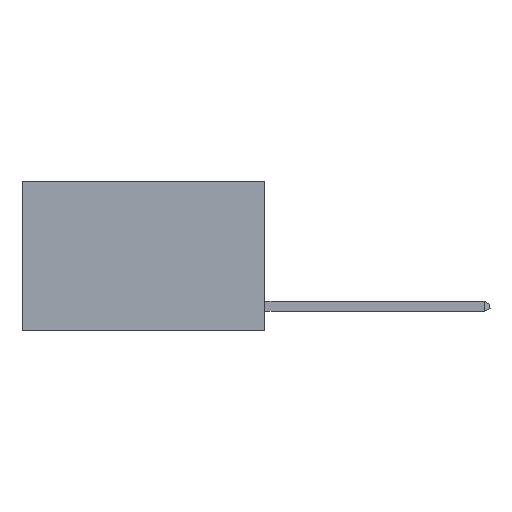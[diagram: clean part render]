
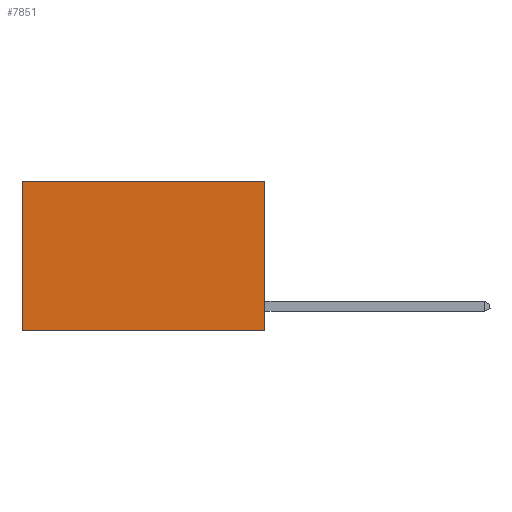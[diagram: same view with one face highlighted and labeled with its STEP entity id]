
A CAD part, left-side view. The second image highlights one B-rep face of the part: STEP entity #7851.
In plain terms, the highlighted planar face has unit normal (-1, 0, 0).
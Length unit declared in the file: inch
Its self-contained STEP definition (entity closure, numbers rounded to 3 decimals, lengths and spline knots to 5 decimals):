
#441 = LINE ( 'NONE', #6357, #4153 ) ;
#710 = ORIENTED_EDGE ( 'NONE', *, *, #3343, .F. ) ;
#729 = ORIENTED_EDGE ( 'NONE', *, *, #4248, .F. ) ;
#936 = CARTESIAN_POINT ( 'NONE',  ( 0.2625, 0., 0. ) ) ;
#1063 = CARTESIAN_POINT ( 'NONE',  ( 0.2625, 0.6, -0.37 ) ) ;
#1352 = DIRECTION ( 'NONE',  ( 0., 0., -1. ) ) ;
#1630 = VERTEX_POINT ( 'NONE', #7407 ) ;
#2320 = VECTOR ( 'NONE', #1352, 39.37008 ) ;
#2380 = DIRECTION ( 'NONE',  ( 0., 0., -1. ) ) ;
#2469 = LINE ( 'NONE', #3936, #7798 ) ;
#2563 = EDGE_CURVE ( 'NONE', #3820, #7483, #6559, .T. ) ;
#3313 = LINE ( 'NONE', #5901, #2320 ) ;
#3343 = EDGE_CURVE ( 'NONE', #3820, #1630, #3313, .T. ) ;
#3380 = CARTESIAN_POINT ( 'NONE',  ( 0.2625, 0., 0. ) ) ;
#3624 = EDGE_CURVE ( 'NONE', #7483, #3974, #441, .T. ) ;
#3820 = VERTEX_POINT ( 'NONE', #936 ) ;
#3936 = CARTESIAN_POINT ( 'NONE',  ( 0.2625, 0., -0.37 ) ) ;
#3944 = DIRECTION ( 'NONE',  ( 0., 1., 0. ) ) ;
#3974 = VERTEX_POINT ( 'NONE', #1063 ) ;
#4153 = VECTOR ( 'NONE', #7576, 39.37008 ) ;
#4248 = EDGE_CURVE ( 'NONE', #1630, #3974, #2469, .T. ) ;
#4838 = PLANE ( 'NONE',  #4973 ) ;
#4973 = AXIS2_PLACEMENT_3D ( 'NONE', #5619, #8109, #2380 ) ;
#5132 = CARTESIAN_POINT ( 'NONE',  ( 0.2625, 0.6, 0. ) ) ;
#5546 = FACE_OUTER_BOUND ( 'NONE', #7777, .T. ) ;
#5619 = CARTESIAN_POINT ( 'NONE',  ( 0.2625, 0., 0. ) ) ;
#5901 = CARTESIAN_POINT ( 'NONE',  ( 0.2625, 0., 0. ) ) ;
#6357 = CARTESIAN_POINT ( 'NONE',  ( 0.2625, 0.6, 0. ) ) ;
#6559 = LINE ( 'NONE', #3380, #6696 ) ;
#6696 = VECTOR ( 'NONE', #3944, 39.37008 ) ;
#6800 = ORIENTED_EDGE ( 'NONE', *, *, #3624, .T. ) ;
#7292 = ORIENTED_EDGE ( 'NONE', *, *, #2563, .T. ) ;
#7407 = CARTESIAN_POINT ( 'NONE',  ( 0.2625, 0., -0.37 ) ) ;
#7483 = VERTEX_POINT ( 'NONE', #5132 ) ;
#7576 = DIRECTION ( 'NONE',  ( 0., 0., -1. ) ) ;
#7777 = EDGE_LOOP ( 'NONE', ( #6800, #729, #710, #7292 ) ) ;
#7798 = VECTOR ( 'NONE', #7936, 39.37008 ) ;
#7851 = ADVANCED_FACE ( 'NONE', ( #5546 ), #4838, .F. ) ;
#7936 = DIRECTION ( 'NONE',  ( 0., 1., 0. ) ) ;
#8109 = DIRECTION ( 'NONE',  ( 1., 0., 0. ) ) ;
